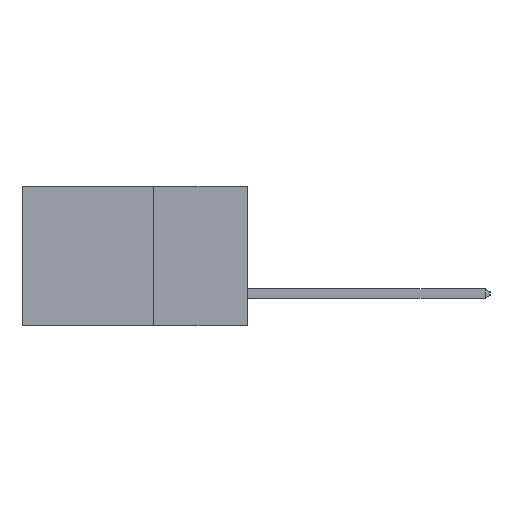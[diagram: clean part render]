
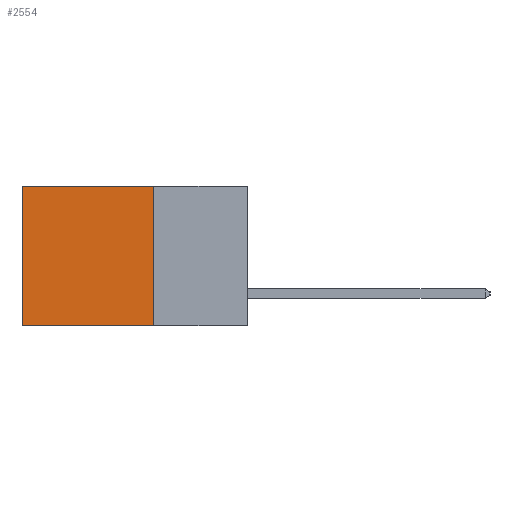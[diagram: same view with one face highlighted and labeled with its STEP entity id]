
A CAD part, left-side view. The second image highlights one B-rep face of the part: STEP entity #2554.
In plain terms, the highlighted planar face has unit normal (-1, 0, 0).
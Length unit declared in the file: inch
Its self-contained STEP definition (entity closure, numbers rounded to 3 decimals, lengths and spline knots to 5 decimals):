
#782 = CARTESIAN_POINT ( 'NONE',  ( 0.2615, 0.25, 0. ) ) ;
#979 = CARTESIAN_POINT ( 'NONE',  ( 0.2615, 0.25, -0.37 ) ) ;
#1345 = VERTEX_POINT ( 'NONE', #979 ) ;
#1614 = FACE_OUTER_BOUND ( 'NONE', #5609, .T. ) ;
#2143 = DIRECTION ( 'NONE',  ( 1., 0., 0. ) ) ;
#2540 = AXIS2_PLACEMENT_3D ( 'NONE', #7348, #2143, #8357 ) ;
#2554 = ADVANCED_FACE ( 'NONE', ( #1614 ), #12652, .F. ) ;
#2652 = EDGE_CURVE ( 'NONE', #9997, #5315, #11938, .T. ) ;
#2754 = EDGE_CURVE ( 'NONE', #1345, #3942, #7661, .T. ) ;
#3306 = CARTESIAN_POINT ( 'NONE',  ( 0.2615, 0.6, -0.37 ) ) ;
#3923 = VECTOR ( 'NONE', #4803, 39.37008 ) ;
#3942 = VERTEX_POINT ( 'NONE', #3306 ) ;
#4462 = VECTOR ( 'NONE', #8144, 39.37008 ) ;
#4616 = CARTESIAN_POINT ( 'NONE',  ( 0.2615, 0.6, -0.37 ) ) ;
#4803 = DIRECTION ( 'NONE',  ( 0., 1., 0. ) ) ;
#5301 = ORIENTED_EDGE ( 'NONE', *, *, #2652, .T. ) ;
#5315 = VERTEX_POINT ( 'NONE', #12221 ) ;
#5609 = EDGE_LOOP ( 'NONE', ( #12326, #6002, #5846, #5301 ) ) ;
#5636 = CARTESIAN_POINT ( 'NONE',  ( 0.2615, 0.25, 0. ) ) ;
#5846 = ORIENTED_EDGE ( 'NONE', *, *, #7120, .F. ) ;
#5935 = VECTOR ( 'NONE', #6812, 39.37008 ) ;
#6002 = ORIENTED_EDGE ( 'NONE', *, *, #2754, .F. ) ;
#6812 = DIRECTION ( 'NONE',  ( 0., 0., -1. ) ) ;
#7120 = EDGE_CURVE ( 'NONE', #9997, #1345, #7371, .T. ) ;
#7316 = EDGE_CURVE ( 'NONE', #5315, #3942, #8696, .T. ) ;
#7348 = CARTESIAN_POINT ( 'NONE',  ( 0.2615, 0.25, -0.37 ) ) ;
#7371 = LINE ( 'NONE', #7809, #4462 ) ;
#7661 = LINE ( 'NONE', #12159, #3923 ) ;
#7809 = CARTESIAN_POINT ( 'NONE',  ( 0.2615, 0.25, -0.37 ) ) ;
#8144 = DIRECTION ( 'NONE',  ( 0., 0., -1. ) ) ;
#8357 = DIRECTION ( 'NONE',  ( 0., 0., -1. ) ) ;
#8696 = LINE ( 'NONE', #4616, #5935 ) ;
#9997 = VERTEX_POINT ( 'NONE', #782 ) ;
#11938 = LINE ( 'NONE', #5636, #12106 ) ;
#12031 = DIRECTION ( 'NONE',  ( 0., 1., 0. ) ) ;
#12106 = VECTOR ( 'NONE', #12031, 39.37008 ) ;
#12159 = CARTESIAN_POINT ( 'NONE',  ( 0.2615, 0.25, -0.37 ) ) ;
#12221 = CARTESIAN_POINT ( 'NONE',  ( 0.2615, 0.6, 0. ) ) ;
#12326 = ORIENTED_EDGE ( 'NONE', *, *, #7316, .T. ) ;
#12652 = PLANE ( 'NONE',  #2540 ) ;
